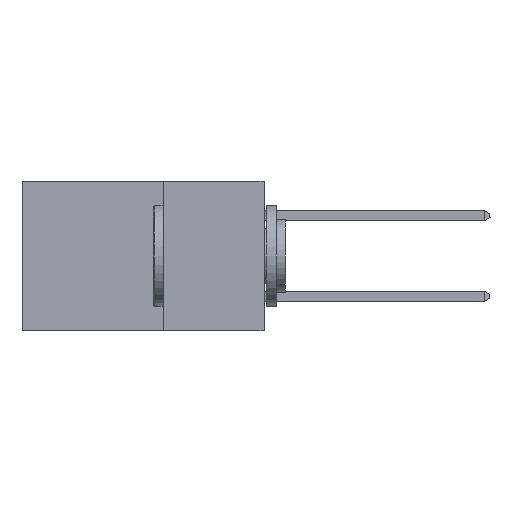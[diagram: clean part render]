
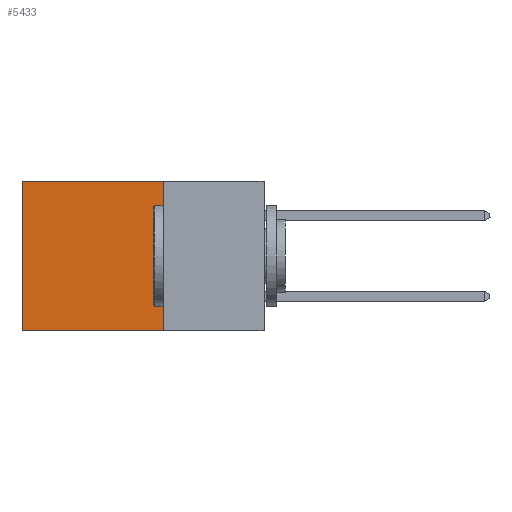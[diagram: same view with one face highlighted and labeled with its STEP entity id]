
A CAD part, left-side view. The second image highlights one B-rep face of the part: STEP entity #5433.
In plain terms, the highlighted planar face has unit normal (-1, 0, 0).
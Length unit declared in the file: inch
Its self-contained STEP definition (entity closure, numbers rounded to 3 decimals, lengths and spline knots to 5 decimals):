
#369 = CARTESIAN_POINT ( 'NONE',  ( 0.298, 0.25, -0.37 ) ) ;
#415 = AXIS2_PLACEMENT_3D ( 'NONE', #14812, #11539, #1486 ) ;
#527 = CARTESIAN_POINT ( 'NONE',  ( 0.298, 0.25, 0. ) ) ;
#1486 = DIRECTION ( 'NONE',  ( 0., 0., -1. ) ) ;
#2698 = VERTEX_POINT ( 'NONE', #10055 ) ;
#2782 = CARTESIAN_POINT ( 'NONE',  ( 0.298, 0.6, 0. ) ) ;
#2790 = VERTEX_POINT ( 'NONE', #6317 ) ;
#3113 = CARTESIAN_POINT ( 'NONE',  ( 0.298, 0.25, 0. ) ) ;
#3941 = VECTOR ( 'NONE', #14804, 39.37008 ) ;
#4957 = VERTEX_POINT ( 'NONE', #13901 ) ;
#5031 = DIRECTION ( 'NONE',  ( 0., 0., -1. ) ) ;
#5433 = ADVANCED_FACE ( 'NONE', ( #16828 ), #21439, .F. ) ;
#5503 = ORIENTED_EDGE ( 'NONE', *, *, #11709, .F. ) ;
#5527 = EDGE_CURVE ( 'NONE', #13377, #2698, #19680, .T. ) ;
#6317 = CARTESIAN_POINT ( 'NONE',  ( 0.298, 0.25, 0. ) ) ;
#7490 = VECTOR ( 'NONE', #12212, 39.37008 ) ;
#8313 = CARTESIAN_POINT ( 'NONE',  ( 0.298, 0.6, 0. ) ) ;
#9817 = ORIENTED_EDGE ( 'NONE', *, *, #19358, .T. ) ;
#10055 = CARTESIAN_POINT ( 'NONE',  ( 0.298, 0.6, -0.37 ) ) ;
#11395 = LINE ( 'NONE', #527, #15819 ) ;
#11539 = DIRECTION ( 'NONE',  ( 1., 0., 0. ) ) ;
#11709 = EDGE_CURVE ( 'NONE', #4957, #2698, #16909, .T. ) ;
#11731 = EDGE_CURVE ( 'NONE', #2790, #4957, #11395, .T. ) ;
#12212 = DIRECTION ( 'NONE',  ( 0., 1., 0. ) ) ;
#12283 = DIRECTION ( 'NONE',  ( 0., 0., -1. ) ) ;
#12481 = ORIENTED_EDGE ( 'NONE', *, *, #11731, .F. ) ;
#12847 = LINE ( 'NONE', #3113, #3941 ) ;
#13377 = VERTEX_POINT ( 'NONE', #2782 ) ;
#13901 = CARTESIAN_POINT ( 'NONE',  ( 0.298, 0.25, -0.37 ) ) ;
#14804 = DIRECTION ( 'NONE',  ( 0., 1., 0. ) ) ;
#14812 = CARTESIAN_POINT ( 'NONE',  ( 0.298, 0.25, 0. ) ) ;
#15819 = VECTOR ( 'NONE', #12283, 39.37008 ) ;
#16271 = ORIENTED_EDGE ( 'NONE', *, *, #5527, .T. ) ;
#16828 = FACE_OUTER_BOUND ( 'NONE', #20358, .T. ) ;
#16909 = LINE ( 'NONE', #369, #7490 ) ;
#19189 = VECTOR ( 'NONE', #5031, 39.37008 ) ;
#19358 = EDGE_CURVE ( 'NONE', #2790, #13377, #12847, .T. ) ;
#19680 = LINE ( 'NONE', #8313, #19189 ) ;
#20358 = EDGE_LOOP ( 'NONE', ( #16271, #5503, #12481, #9817 ) ) ;
#21439 = PLANE ( 'NONE',  #415 ) ;
